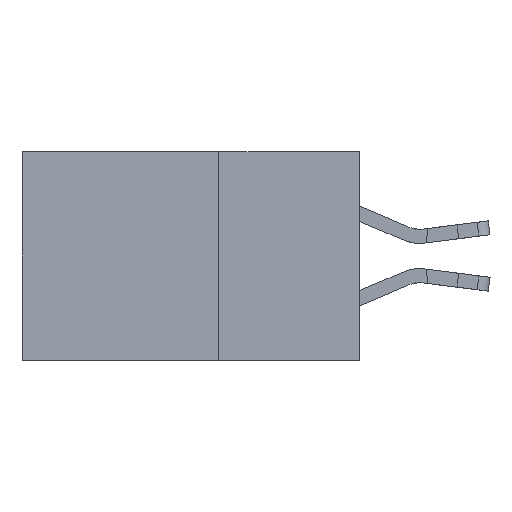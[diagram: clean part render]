
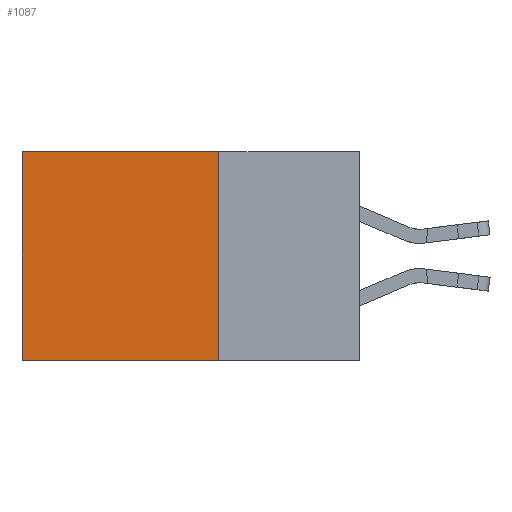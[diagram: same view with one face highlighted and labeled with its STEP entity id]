
A CAD part, left-side view. The second image highlights one B-rep face of the part: STEP entity #1087.
In plain terms, the highlighted planar face has unit normal (-1, 0, 0).
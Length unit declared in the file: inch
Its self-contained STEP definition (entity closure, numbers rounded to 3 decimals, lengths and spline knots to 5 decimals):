
#327 = LINE ( 'NONE', #17905, #7909 ) ;
#588 = CARTESIAN_POINT ( 'NONE',  ( 0.2875, 0.6, -0.37 ) ) ;
#641 = EDGE_CURVE ( 'NONE', #7862, #8011, #21590, .T. ) ;
#1060 = FACE_OUTER_BOUND ( 'NONE', #3398, .T. ) ;
#1087 = ADVANCED_FACE ( 'NONE', ( #1060 ), #10279, .F. ) ;
#1212 = VERTEX_POINT ( 'NONE', #16706 ) ;
#2663 = ORIENTED_EDGE ( 'NONE', *, *, #12627, .T. ) ;
#3398 = EDGE_LOOP ( 'NONE', ( #25102, #24494, #7038, #2663 ) ) ;
#4101 = DIRECTION ( 'NONE',  ( 0., 1., 0. ) ) ;
#6005 = CARTESIAN_POINT ( 'NONE',  ( 0.2875, 0.25, 0. ) ) ;
#6210 = VECTOR ( 'NONE', #10194, 39.37008 ) ;
#6229 = CARTESIAN_POINT ( 'NONE',  ( 0.2875, 0.25, -0.37 ) ) ;
#6785 = VECTOR ( 'NONE', #4101, 39.37008 ) ;
#7038 = ORIENTED_EDGE ( 'NONE', *, *, #16758, .F. ) ;
#7219 = VERTEX_POINT ( 'NONE', #21687 ) ;
#7345 = LINE ( 'NONE', #19966, #22460 ) ;
#7862 = VERTEX_POINT ( 'NONE', #11722 ) ;
#7909 = VECTOR ( 'NONE', #17743, 39.37008 ) ;
#8011 = VERTEX_POINT ( 'NONE', #588 ) ;
#10194 = DIRECTION ( 'NONE',  ( 0., 0., -1. ) ) ;
#10279 = PLANE ( 'NONE',  #21728 ) ;
#11722 = CARTESIAN_POINT ( 'NONE',  ( 0.2875, 0.25, -0.37 ) ) ;
#11973 = DIRECTION ( 'NONE',  ( 0., 0., -1. ) ) ;
#12473 = LINE ( 'NONE', #20146, #6210 ) ;
#12627 = EDGE_CURVE ( 'NONE', #1212, #7219, #7345, .T. ) ;
#13852 = DIRECTION ( 'NONE',  ( 0., 1., 0. ) ) ;
#16099 = DIRECTION ( 'NONE',  ( 1., 0., 0. ) ) ;
#16706 = CARTESIAN_POINT ( 'NONE',  ( 0.2875, 0.25, 0. ) ) ;
#16758 = EDGE_CURVE ( 'NONE', #1212, #7862, #12473, .T. ) ;
#17743 = DIRECTION ( 'NONE',  ( 0., 0., -1. ) ) ;
#17905 = CARTESIAN_POINT ( 'NONE',  ( 0.2875, 0.6, 0. ) ) ;
#19966 = CARTESIAN_POINT ( 'NONE',  ( 0.2875, 0.25, 0. ) ) ;
#20080 = EDGE_CURVE ( 'NONE', #7219, #8011, #327, .T. ) ;
#20146 = CARTESIAN_POINT ( 'NONE',  ( 0.2875, 0.25, 0. ) ) ;
#21590 = LINE ( 'NONE', #6229, #6785 ) ;
#21687 = CARTESIAN_POINT ( 'NONE',  ( 0.2875, 0.6, 0. ) ) ;
#21728 = AXIS2_PLACEMENT_3D ( 'NONE', #6005, #16099, #11973 ) ;
#22460 = VECTOR ( 'NONE', #13852, 39.37008 ) ;
#24494 = ORIENTED_EDGE ( 'NONE', *, *, #641, .F. ) ;
#25102 = ORIENTED_EDGE ( 'NONE', *, *, #20080, .T. ) ;
